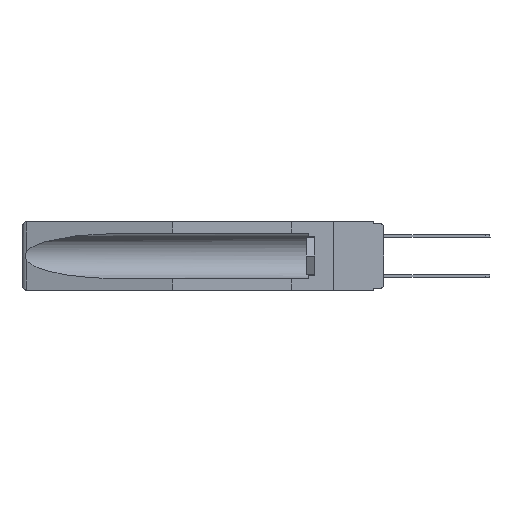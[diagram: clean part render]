
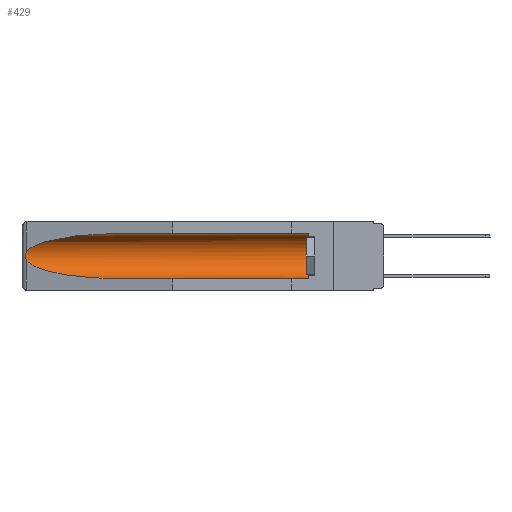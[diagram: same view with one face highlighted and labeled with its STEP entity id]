
A CAD part, left-side view. The second image highlights one B-rep face of the part: STEP entity #429.
In plain terms, the highlighted cylindrical face has radius 2.857 mm (diameter 5.715 mm), a partial arc.
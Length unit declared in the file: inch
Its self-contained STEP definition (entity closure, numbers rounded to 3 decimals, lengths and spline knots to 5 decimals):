
#429 = ADVANCED_FACE ( 'NONE', ( #3154 ), #8447, .F. ) ;
#947 = EDGE_CURVE ( 'NONE', #23023, #20151, #13115, .T. ) ;
#1024 = CARTESIAN_POINT ( 'NONE',  ( 0.25451, 1.48313, -0.09465 ) ) ;
#1081 = ORIENTED_EDGE ( 'NONE', *, *, #8467, .T. ) ;
#1209 = VERTEX_POINT ( 'NONE', #2087 ) ;
#2087 = CARTESIAN_POINT ( 'NONE',  ( 0.26537, 1.52718, -0.14972 ) ) ;
#3154 = FACE_OUTER_BOUND ( 'NONE', #17337, .T. ) ;
#3271 = ORIENTED_EDGE ( 'NONE', *, *, #24534, .T. ) ;
#3528 = CARTESIAN_POINT ( 'NONE',  ( 0.26537, 1.52718, -0.14972 ) ) ;
#3552 = CIRCLE ( 'NONE', #22897, 0.1125 ) ;
#3626 = CARTESIAN_POINT ( 'NONE',  ( 0.155, 0.126, -0.1715 ) ) ;
#3984 = VECTOR ( 'NONE', #27265, 39.37008 ) ;
#5485 = DIRECTION ( 'NONE',  ( 0., -1., 0. ) ) ;
#6786 = CARTESIAN_POINT ( 'NONE',  ( 0.155, 0.126, -0.284 ) ) ;
#7209 = CARTESIAN_POINT ( 'NONE',  ( 0.155, 1.07973, -0.059 ) ) ;
#7258 = EDGE_CURVE ( 'NONE', #14662, #1209, #20888, .T. ) ;
#7498 = EDGE_CURVE ( 'NONE', #12447, #20151, #10637, .T. ) ;
#7582 = CARTESIAN_POINT ( 'NONE',  ( 0.155, 1.07973, -0.284 ) ) ;
#7617 = DIRECTION ( 'NONE',  ( 0., 0., 1. ) ) ;
#8086 = DIRECTION ( 'NONE',  ( 0., 1., 0. ) ) ;
#8447 = CYLINDRICAL_SURFACE ( 'NONE', #23222, 0.1125 ) ;
#8467 = EDGE_CURVE ( 'NONE', #1209, #23023, #24630, .T. ) ;
#8819 = CARTESIAN_POINT ( 'NONE',  ( 0.155, 0.126, -0.059 ) ) ;
#9707 = VECTOR ( 'NONE', #8086, 39.37008 ) ;
#9755 = CARTESIAN_POINT ( 'NONE',  ( 0.26537, 1.52718, -0.19328 ) ) ;
#9939 = CARTESIAN_POINT ( 'NONE',  ( 0.26655, 1.53094, -0.18657 ) ) ;
#10606 = CARTESIAN_POINT ( 'NONE',  ( 0.155, 1.07973, -0.284 ) ) ;
#10637 = LINE ( 'NONE', #12329, #3984 ) ;
#11896 = CARTESIAN_POINT ( 'NONE',  ( 0.2675, 1.53308, -0.17534 ) ) ;
#11975 = CARTESIAN_POINT ( 'NONE',  ( 0.155, -0.30754, -0.1715 ) ) ;
#12183 = CARTESIAN_POINT ( 'NONE',  ( 0.2673, 1.53269, -0.17917 ) ) ;
#12329 = CARTESIAN_POINT ( 'NONE',  ( 0.155, -0.30754, -0.284 ) ) ;
#12447 = VERTEX_POINT ( 'NONE', #6786 ) ;
#12668 = CARTESIAN_POINT ( 'NONE',  ( 0.25451, 1.48313, -0.24835 ) ) ;
#12669 = CARTESIAN_POINT ( 'NONE',  ( 0.26537, 1.52718, -0.19328 ) ) ;
#12711 = DIRECTION ( 'NONE',  ( 0., 1., 0. ) ) ;
#13115 =( BOUNDED_CURVE ( )  B_SPLINE_CURVE ( 3, ( #22960, #12668, #27522, #10606 ),
 .UNSPECIFIED., .F., .F. ) 
 B_SPLINE_CURVE_WITH_KNOTS ( ( 4, 4 ),
 ( 0.1948, 1.5708 ),
 .UNSPECIFIED. ) 
 CURVE ( )  GEOMETRIC_REPRESENTATION_ITEM ( )  RATIONAL_B_SPLINE_CURVE ( ( 1., 0.848, 0.848, 1. ) ) 
 REPRESENTATION_ITEM ( '' )  );
#14209 = CARTESIAN_POINT ( 'NONE',  ( 0.2673, 1.5327, -0.16383 ) ) ;
#14309 = CARTESIAN_POINT ( 'NONE',  ( 0.155, -0.30754, -0.059 ) ) ;
#14662 = VERTEX_POINT ( 'NONE', #7209 ) ;
#15349 = LINE ( 'NONE', #14309, #9707 ) ;
#16284 = ORIENTED_EDGE ( 'NONE', *, *, #947, .T. ) ;
#17337 = EDGE_LOOP ( 'NONE', ( #27298, #1081, #16284, #19033, #3271, #25292 ) ) ;
#17812 = CARTESIAN_POINT ( 'NONE',  ( 0.155, 1.07973, -0.059 ) ) ;
#19033 = ORIENTED_EDGE ( 'NONE', *, *, #7498, .F. ) ;
#20151 = VERTEX_POINT ( 'NONE', #7582 ) ;
#20706 = CARTESIAN_POINT ( 'NONE',  ( 0.26654, 1.53092, -0.15636 ) ) ;
#20888 =( BOUNDED_CURVE ( )  B_SPLINE_CURVE ( 3, ( #17812, #22191, #1024, #22107 ),
 .UNSPECIFIED., .F., .F. ) 
 B_SPLINE_CURVE_WITH_KNOTS ( ( 4, 4 ),
 ( 4.71239, 6.08839 ),
 .UNSPECIFIED. ) 
 CURVE ( )  GEOMETRIC_REPRESENTATION_ITEM ( )  RATIONAL_B_SPLINE_CURVE ( ( 1., 0.848, 0.848, 1. ) ) 
 REPRESENTATION_ITEM ( '' )  );
#21627 = EDGE_CURVE ( 'NONE', #24797, #14662, #15349, .T. ) ;
#22107 = CARTESIAN_POINT ( 'NONE',  ( 0.26537, 1.52718, -0.14972 ) ) ;
#22191 = CARTESIAN_POINT ( 'NONE',  ( 0.21114, 1.30732, -0.059 ) ) ;
#22832 = CARTESIAN_POINT ( 'NONE',  ( 0.26597, 1.52961, -0.15275 ) ) ;
#22897 = AXIS2_PLACEMENT_3D ( 'NONE', #3626, #5485, #7617 ) ;
#22960 = CARTESIAN_POINT ( 'NONE',  ( 0.26537, 1.52718, -0.19328 ) ) ;
#23023 = VERTEX_POINT ( 'NONE', #12669 ) ;
#23222 = AXIS2_PLACEMENT_3D ( 'NONE', #11975, #12711, #23267 ) ;
#23267 = DIRECTION ( 'NONE',  ( 0., 0., 1. ) ) ;
#24534 = EDGE_CURVE ( 'NONE', #12447, #24797, #3552, .T. ) ;
#24630 = B_SPLINE_CURVE_WITH_KNOTS ( 'NONE', 3,
 ( #3528, #22832, #20706, #14209, #27119, #11896, #12183, #9939, #24785, #9755 ),
 .UNSPECIFIED., .F., .F.,
 ( 4, 2, 2, 2, 4 ),
 ( 0., 0.00029, 0.00058, 0.00087, 0.00117 ),
 .UNSPECIFIED. ) ;
#24785 = CARTESIAN_POINT ( 'NONE',  ( 0.26597, 1.5296, -0.19026 ) ) ;
#24797 = VERTEX_POINT ( 'NONE', #8819 ) ;
#25292 = ORIENTED_EDGE ( 'NONE', *, *, #21627, .T. ) ;
#27119 = CARTESIAN_POINT ( 'NONE',  ( 0.2675, 1.53308, -0.16763 ) ) ;
#27265 = DIRECTION ( 'NONE',  ( 0., 1., 0. ) ) ;
#27298 = ORIENTED_EDGE ( 'NONE', *, *, #7258, .T. ) ;
#27522 = CARTESIAN_POINT ( 'NONE',  ( 0.21114, 1.30732, -0.284 ) ) ;
